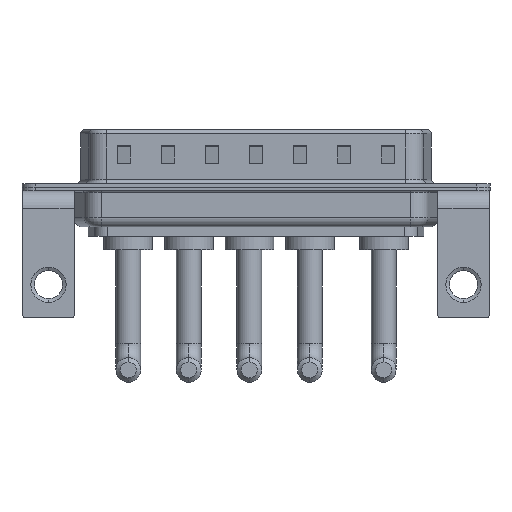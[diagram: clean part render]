
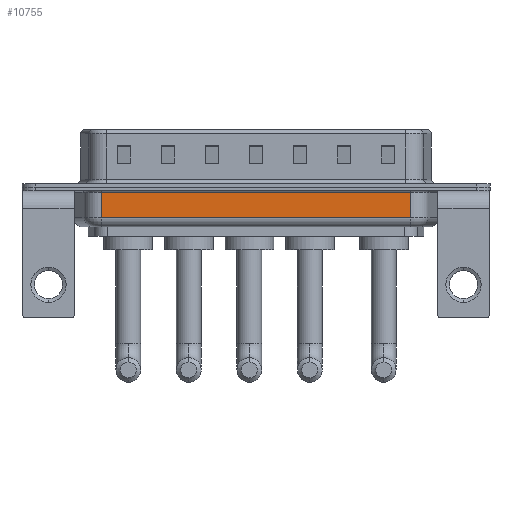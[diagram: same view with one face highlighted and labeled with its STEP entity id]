
A CAD part, front view. The second image highlights one B-rep face of the part: STEP entity #10755.
In plain terms, the highlighted planar face has unit normal (0, -1, 0).
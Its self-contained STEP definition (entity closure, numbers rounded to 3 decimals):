
#19 = LINE ( 'NONE', #9440, #12858 ) ;
#35 = DIRECTION ( 'NONE',  ( 0., 0., 1. ) ) ;
#182 = VERTEX_POINT ( 'NONE', #8618 ) ;
#1536 = EDGE_LOOP ( 'NONE', ( #8364, #7042, #9430, #6299 ) ) ;
#1732 = EDGE_CURVE ( 'NONE', #10051, #1851, #4771, .T. ) ;
#1851 = VERTEX_POINT ( 'NONE', #8530 ) ;
#2075 = FACE_OUTER_BOUND ( 'NONE', #1536, .T. ) ;
#2538 = DIRECTION ( 'NONE',  ( 0., 0., 1. ) ) ;
#3490 = EDGE_CURVE ( 'NONE', #1851, #11969, #9361, .T. ) ;
#3500 = EDGE_CURVE ( 'NONE', #182, #11969, #19, .T. ) ;
#3751 = CARTESIAN_POINT ( 'NONE',  ( 6.006, -5.35, -0.65 ) ) ;
#4771 = LINE ( 'NONE', #9606, #5683 ) ;
#4825 = DIRECTION ( 'NONE',  ( -1., 0., 0. ) ) ;
#5425 = PLANE ( 'NONE',  #13569 ) ;
#5683 = VECTOR ( 'NONE', #35, 1000. ) ;
#6082 = CARTESIAN_POINT ( 'NONE',  ( 6.006, -5.35, -0.65 ) ) ;
#6299 = ORIENTED_EDGE ( 'NONE', *, *, #3490, .T. ) ;
#6967 = VECTOR ( 'NONE', #11796, 1000. ) ;
#7042 = ORIENTED_EDGE ( 'NONE', *, *, #11294, .T. ) ;
#7884 = CARTESIAN_POINT ( 'NONE',  ( 6.006, -5.35, -4.5 ) ) ;
#8364 = ORIENTED_EDGE ( 'NONE', *, *, #3500, .F. ) ;
#8530 = CARTESIAN_POINT ( 'NONE',  ( 41.044, -5.35, -0.65 ) ) ;
#8618 = CARTESIAN_POINT ( 'NONE',  ( 6.006, -5.35, -3.5 ) ) ;
#9361 = LINE ( 'NONE', #3751, #14567 ) ;
#9430 = ORIENTED_EDGE ( 'NONE', *, *, #1732, .T. ) ;
#9440 = CARTESIAN_POINT ( 'NONE',  ( 6.006, -5.35, -4.5 ) ) ;
#9606 = CARTESIAN_POINT ( 'NONE',  ( 41.044, -5.35, -4.5 ) ) ;
#10051 = VERTEX_POINT ( 'NONE', #13178 ) ;
#10502 = CARTESIAN_POINT ( 'NONE',  ( 6.006, -5.35, -3.5 ) ) ;
#10755 = ADVANCED_FACE ( 'NONE', ( #2075 ), #5425, .F. ) ;
#11294 = EDGE_CURVE ( 'NONE', #182, #10051, #12795, .T. ) ;
#11513 = DIRECTION ( 'NONE',  ( 0., 0., 1. ) ) ;
#11796 = DIRECTION ( 'NONE',  ( 1., 0., 0. ) ) ;
#11969 = VERTEX_POINT ( 'NONE', #6082 ) ;
#12355 = DIRECTION ( 'NONE',  ( 0., 1., 0. ) ) ;
#12795 = LINE ( 'NONE', #10502, #6967 ) ;
#12858 = VECTOR ( 'NONE', #2538, 1000. ) ;
#13178 = CARTESIAN_POINT ( 'NONE',  ( 41.044, -5.35, -3.5 ) ) ;
#13569 = AXIS2_PLACEMENT_3D ( 'NONE', #7884, #12355, #11513 ) ;
#14567 = VECTOR ( 'NONE', #4825, 1000. ) ;
